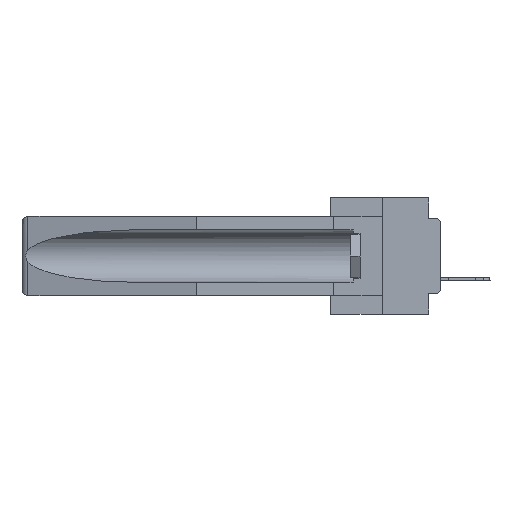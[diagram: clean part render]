
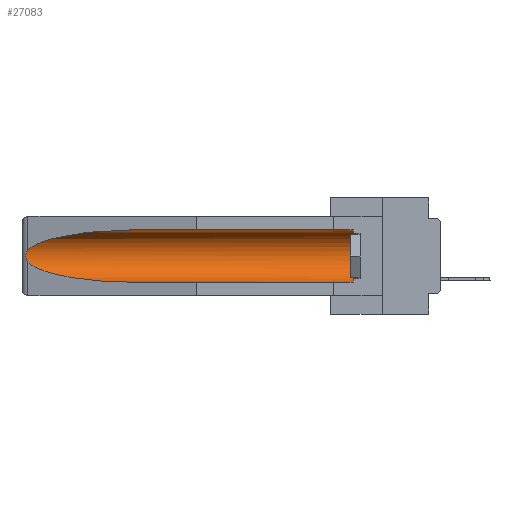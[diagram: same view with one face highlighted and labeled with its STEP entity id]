
A CAD part, left-side view. The second image highlights one B-rep face of the part: STEP entity #27083.
In plain terms, the highlighted cylindrical face has radius 2.857 mm (diameter 5.715 mm), a partial arc.
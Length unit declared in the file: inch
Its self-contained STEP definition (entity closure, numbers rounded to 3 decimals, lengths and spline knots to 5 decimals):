
#144 = VECTOR ( 'NONE', #29547, 39.37008 ) ;
#146 = AXIS2_PLACEMENT_3D ( 'NONE', #24537, #13569, #27717 ) ;
#196 = CARTESIAN_POINT ( 'NONE',  ( 0.155, 1.07973, -0.059 ) ) ;
#2357 =( BOUNDED_CURVE ( )  B_SPLINE_CURVE ( 3, ( #4191, #5055, #15478, #21064 ),
 .UNSPECIFIED., .F., .F. ) 
 B_SPLINE_CURVE_WITH_KNOTS ( ( 4, 4 ),
 ( 4.71239, 6.08839 ),
 .UNSPECIFIED. ) 
 CURVE ( )  GEOMETRIC_REPRESENTATION_ITEM ( )  RATIONAL_B_SPLINE_CURVE ( ( 1., 0.848, 0.848, 1. ) ) 
 REPRESENTATION_ITEM ( '' )  );
#3501 = CARTESIAN_POINT ( 'NONE',  ( 0.26537, 1.52718, -0.19328 ) ) ;
#3788 = CARTESIAN_POINT ( 'NONE',  ( 0.25451, 1.48313, -0.24835 ) ) ;
#4191 = CARTESIAN_POINT ( 'NONE',  ( 0.155, 1.07973, -0.059 ) ) ;
#5055 = CARTESIAN_POINT ( 'NONE',  ( 0.21114, 1.30732, -0.059 ) ) ;
#5399 = LINE ( 'NONE', #34940, #144 ) ;
#5891 = EDGE_CURVE ( 'NONE', #30258, #19876, #2357, .T. ) ;
#6339 = LINE ( 'NONE', #20994, #19924 ) ;
#6479 = CARTESIAN_POINT ( 'NONE',  ( 0.26537, 1.52718, -0.19328 ) ) ;
#6685 = CARTESIAN_POINT ( 'NONE',  ( 0.155, 0.126, -0.059 ) ) ;
#6960 = CARTESIAN_POINT ( 'NONE',  ( 0.26537, 1.52718, -0.14972 ) ) ;
#8690 = CYLINDRICAL_SURFACE ( 'NONE', #25356, 0.1125 ) ;
#8735 = EDGE_CURVE ( 'NONE', #28974, #23043, #6339, .T. ) ;
#8876 = CARTESIAN_POINT ( 'NONE',  ( 0.26655, 1.53094, -0.18657 ) ) ;
#9300 = EDGE_CURVE ( 'NONE', #28142, #23043, #34410, .T. ) ;
#10251 = EDGE_CURVE ( 'NONE', #35609, #30258, #5399, .T. ) ;
#10430 = ORIENTED_EDGE ( 'NONE', *, *, #10251, .T. ) ;
#11584 = CARTESIAN_POINT ( 'NONE',  ( 0.2675, 1.53308, -0.16763 ) ) ;
#12387 = CARTESIAN_POINT ( 'NONE',  ( 0.21114, 1.30732, -0.284 ) ) ;
#13569 = DIRECTION ( 'NONE',  ( 0., -1., 0. ) ) ;
#15478 = CARTESIAN_POINT ( 'NONE',  ( 0.25451, 1.48313, -0.09465 ) ) ;
#15543 = EDGE_CURVE ( 'NONE', #19876, #28142, #36009, .T. ) ;
#15557 = CARTESIAN_POINT ( 'NONE',  ( 0.155, 1.07973, -0.284 ) ) ;
#16143 = ORIENTED_EDGE ( 'NONE', *, *, #28913, .T. ) ;
#18190 = ORIENTED_EDGE ( 'NONE', *, *, #5891, .T. ) ;
#18333 = ORIENTED_EDGE ( 'NONE', *, *, #8735, .F. ) ;
#18694 = DIRECTION ( 'NONE',  ( 0., 0., 1. ) ) ;
#19876 = VERTEX_POINT ( 'NONE', #6960 ) ;
#19924 = VECTOR ( 'NONE', #29714, 39.37008 ) ;
#20258 = CARTESIAN_POINT ( 'NONE',  ( 0.26597, 1.5296, -0.19026 ) ) ;
#20791 = ORIENTED_EDGE ( 'NONE', *, *, #15543, .T. ) ;
#20994 = CARTESIAN_POINT ( 'NONE',  ( 0.155, -0.30754, -0.284 ) ) ;
#21064 = CARTESIAN_POINT ( 'NONE',  ( 0.26537, 1.52718, -0.14972 ) ) ;
#21416 = CARTESIAN_POINT ( 'NONE',  ( 0.26537, 1.52718, -0.19328 ) ) ;
#22652 = EDGE_LOOP ( 'NONE', ( #18190, #20791, #29469, #18333, #16143, #10430 ) ) ;
#22698 = CARTESIAN_POINT ( 'NONE',  ( 0.26537, 1.52718, -0.14972 ) ) ;
#22816 = CARTESIAN_POINT ( 'NONE',  ( 0.2673, 1.5327, -0.16383 ) ) ;
#23043 = VERTEX_POINT ( 'NONE', #24760 ) ;
#24537 = CARTESIAN_POINT ( 'NONE',  ( 0.155, 0.126, -0.1715 ) ) ;
#24760 = CARTESIAN_POINT ( 'NONE',  ( 0.155, 1.07973, -0.284 ) ) ;
#25356 = AXIS2_PLACEMENT_3D ( 'NONE', #29851, #32668, #18694 ) ;
#26504 = CIRCLE ( 'NONE', #146, 0.1125 ) ;
#27083 = ADVANCED_FACE ( 'NONE', ( #35935 ), #8690, .F. ) ;
#27717 = DIRECTION ( 'NONE',  ( 0., 0., 1. ) ) ;
#28142 = VERTEX_POINT ( 'NONE', #21416 ) ;
#28328 = CARTESIAN_POINT ( 'NONE',  ( 0.26597, 1.52961, -0.15275 ) ) ;
#28455 = CARTESIAN_POINT ( 'NONE',  ( 0.26654, 1.53092, -0.15636 ) ) ;
#28913 = EDGE_CURVE ( 'NONE', #28974, #35609, #26504, .T. ) ;
#28974 = VERTEX_POINT ( 'NONE', #36216 ) ;
#29469 = ORIENTED_EDGE ( 'NONE', *, *, #9300, .T. ) ;
#29547 = DIRECTION ( 'NONE',  ( 0., 1., 0. ) ) ;
#29714 = DIRECTION ( 'NONE',  ( 0., 1., 0. ) ) ;
#29851 = CARTESIAN_POINT ( 'NONE',  ( 0.155, -0.30754, -0.1715 ) ) ;
#30258 = VERTEX_POINT ( 'NONE', #196 ) ;
#31168 = CARTESIAN_POINT ( 'NONE',  ( 0.2673, 1.53269, -0.17917 ) ) ;
#31523 = CARTESIAN_POINT ( 'NONE',  ( 0.2675, 1.53308, -0.17534 ) ) ;
#32668 = DIRECTION ( 'NONE',  ( 0., 1., 0. ) ) ;
#34410 =( BOUNDED_CURVE ( )  B_SPLINE_CURVE ( 3, ( #6479, #3788, #12387, #15557 ),
 .UNSPECIFIED., .F., .T. ) 
 B_SPLINE_CURVE_WITH_KNOTS ( ( 4, 4 ),
 ( 0.1948, 1.5708 ),
 .UNSPECIFIED. ) 
 CURVE ( )  GEOMETRIC_REPRESENTATION_ITEM ( )  RATIONAL_B_SPLINE_CURVE ( ( 1., 0.848, 0.848, 1. ) ) 
 REPRESENTATION_ITEM ( '' )  );
#34940 = CARTESIAN_POINT ( 'NONE',  ( 0.155, -0.30754, -0.059 ) ) ;
#35609 = VERTEX_POINT ( 'NONE', #6685 ) ;
#35935 = FACE_OUTER_BOUND ( 'NONE', #22652, .T. ) ;
#36009 = B_SPLINE_CURVE_WITH_KNOTS ( 'NONE', 3,
 ( #22698, #28328, #28455, #22816, #11584, #31523, #31168, #8876, #20258, #3501 ),
 .UNSPECIFIED., .F., .F.,
 ( 4, 2, 2, 2, 4 ),
 ( 0., 0.00029, 0.00058, 0.00087, 0.00117 ),
 .UNSPECIFIED. ) ;
#36216 = CARTESIAN_POINT ( 'NONE',  ( 0.155, 0.126, -0.284 ) ) ;
